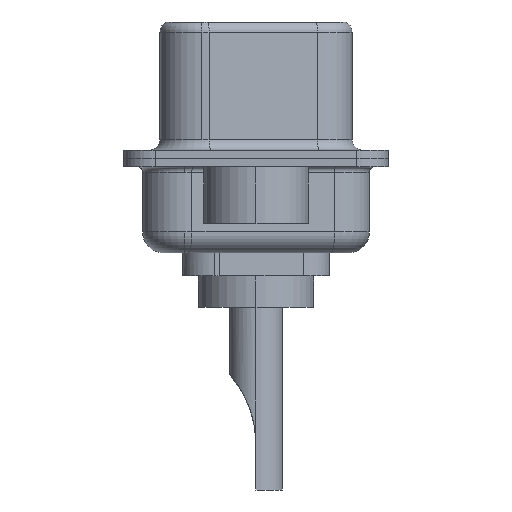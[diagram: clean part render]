
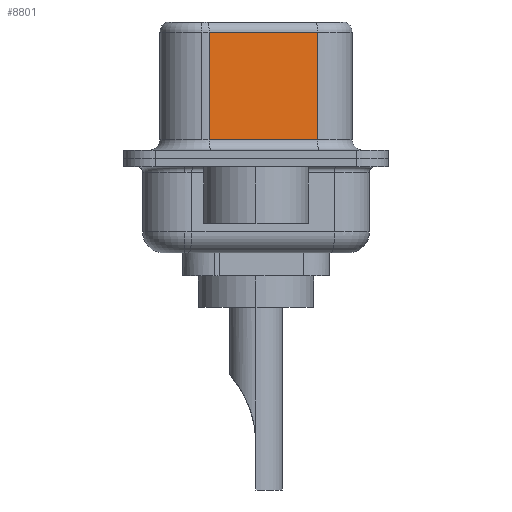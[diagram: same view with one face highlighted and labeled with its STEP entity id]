
A CAD part, left-side view. The second image highlights one B-rep face of the part: STEP entity #8801.
In plain terms, the highlighted planar face has unit normal (-0.985, -0.174, 0).
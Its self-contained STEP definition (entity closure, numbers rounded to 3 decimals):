
#1 = ORIENTED_EDGE ( 'NONE', *, *, #1086, .T. ) ;
#149 = ORIENTED_EDGE ( 'NONE', *, *, #2659, .T. ) ;
#1064 = CARTESIAN_POINT ( 'NONE',  ( 3.655, 2.233, 6.02 ) ) ;
#1086 = EDGE_CURVE ( 'NONE', #4655, #12188, #8881, .T. ) ;
#2524 = EDGE_CURVE ( 'NONE', #12188, #14523, #8885, .T. ) ;
#2632 = EDGE_CURVE ( 'NONE', #10185, #14523, #11007, .T. ) ;
#2659 = EDGE_CURVE ( 'NONE', #10185, #4655, #13777, .T. ) ;
#3176 = ORIENTED_EDGE ( 'NONE', *, *, #2524, .T. ) ;
#3718 = VECTOR ( 'NONE', #3811, 1000. ) ;
#3811 = DIRECTION ( 'NONE',  ( -0.174, 0.985, 0. ) ) ;
#4520 = DIRECTION ( 'NONE',  ( 0.174, -0.985, 0. ) ) ;
#4655 = VERTEX_POINT ( 'NONE', #1064 ) ;
#4895 = DIRECTION ( 'NONE',  ( 0., 0., -1. ) ) ;
#5312 = DIRECTION ( 'NONE',  ( 0., 0., -1. ) ) ;
#5340 = VECTOR ( 'NONE', #4520, 1000. ) ;
#5629 = AXIS2_PLACEMENT_3D ( 'NONE', #13940, #13843, #13784 ) ;
#5705 = ORIENTED_EDGE ( 'NONE', *, *, #2632, .F. ) ;
#5720 = VECTOR ( 'NONE', #5312, 1000. ) ;
#7633 = VECTOR ( 'NONE', #4895, 1000. ) ;
#7737 = CARTESIAN_POINT ( 'NONE',  ( 4.565, -2.927, 6.02 ) ) ;
#8377 = CARTESIAN_POINT ( 'NONE',  ( 4.565, -2.927, 6.02 ) ) ;
#8549 = PLANE ( 'NONE',  #5629 ) ;
#8801 = ADVANCED_FACE ( 'NONE', ( #14786 ), #8549, .F. ) ;
#8881 = LINE ( 'NONE', #14454, #5720 ) ;
#8885 = LINE ( 'NONE', #11288, #5340 ) ;
#8924 = EDGE_LOOP ( 'NONE', ( #5705, #149, #1, #3176 ) ) ;
#10185 = VERTEX_POINT ( 'NONE', #7737 ) ;
#11007 = LINE ( 'NONE', #13965, #7633 ) ;
#11288 = CARTESIAN_POINT ( 'NONE',  ( 4.565, -2.927, 0.9 ) ) ;
#12188 = VERTEX_POINT ( 'NONE', #12237 ) ;
#12237 = CARTESIAN_POINT ( 'NONE',  ( 3.655, 2.233, 0.9 ) ) ;
#13777 = LINE ( 'NONE', #8377, #3718 ) ;
#13784 = DIRECTION ( 'NONE',  ( -0.174, 0.985, 0. ) ) ;
#13843 = DIRECTION ( 'NONE',  ( 0.985, 0.174, 0. ) ) ;
#13940 = CARTESIAN_POINT ( 'NONE',  ( 4.565, -2.927, 6.52 ) ) ;
#13965 = CARTESIAN_POINT ( 'NONE',  ( 4.565, -2.927, 6.52 ) ) ;
#14454 = CARTESIAN_POINT ( 'NONE',  ( 3.655, 2.233, 6.52 ) ) ;
#14523 = VERTEX_POINT ( 'NONE', #15868 ) ;
#14786 = FACE_OUTER_BOUND ( 'NONE', #8924, .T. ) ;
#15868 = CARTESIAN_POINT ( 'NONE',  ( 4.565, -2.927, 0.9 ) ) ;
